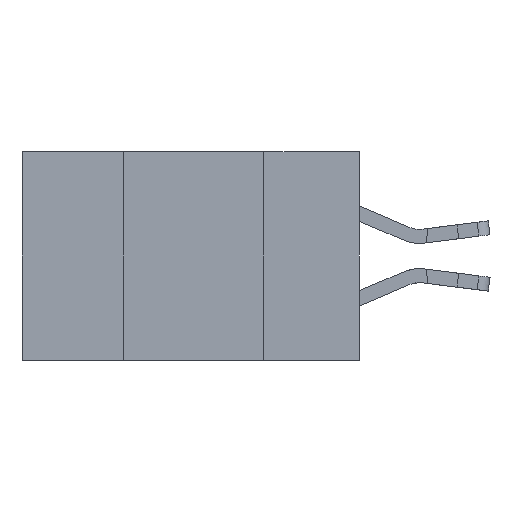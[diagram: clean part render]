
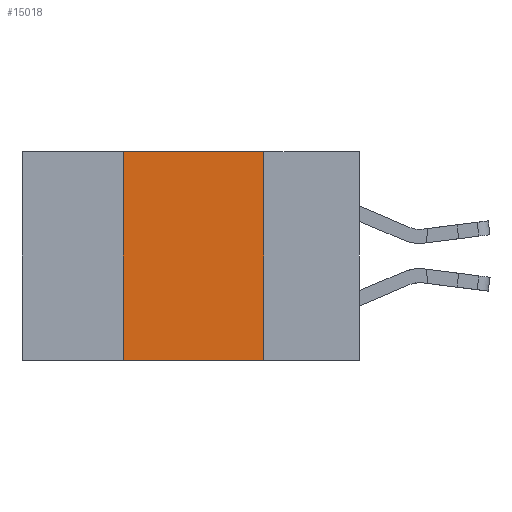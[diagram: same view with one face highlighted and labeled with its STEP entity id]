
A CAD part, left-side view. The second image highlights one B-rep face of the part: STEP entity #15018.
In plain terms, the highlighted planar face has unit normal (-1, 0, 0).
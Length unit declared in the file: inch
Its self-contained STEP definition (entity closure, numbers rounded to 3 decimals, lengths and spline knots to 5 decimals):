
#523 = AXIS2_PLACEMENT_3D ( 'NONE', #17458, #7223, #19113 ) ;
#572 = VERTEX_POINT ( 'NONE', #14570 ) ;
#1263 = CARTESIAN_POINT ( 'NONE',  ( 0., 0.17, 0. ) ) ;
#1978 = FACE_OUTER_BOUND ( 'NONE', #13921, .T. ) ;
#2129 = CARTESIAN_POINT ( 'NONE',  ( 0., 0.42, 0. ) ) ;
#2309 = CARTESIAN_POINT ( 'NONE',  ( 0., 0.42, 0. ) ) ;
#2431 = VECTOR ( 'NONE', #11048, 39.37008 ) ;
#2872 = VECTOR ( 'NONE', #20159, 39.37008 ) ;
#3584 = CARTESIAN_POINT ( 'NONE',  ( 0., 0.6, 0. ) ) ;
#5755 = VERTEX_POINT ( 'NONE', #6337 ) ;
#6337 = CARTESIAN_POINT ( 'NONE',  ( 0., 0.17, 0. ) ) ;
#6948 = DIRECTION ( 'NONE',  ( 0., -1., 0. ) ) ;
#7058 = LINE ( 'NONE', #3584, #20064 ) ;
#7223 = DIRECTION ( 'NONE',  ( 1., 0., 0. ) ) ;
#8259 = VERTEX_POINT ( 'NONE', #2129 ) ;
#8602 = EDGE_CURVE ( 'NONE', #5755, #572, #12103, .T. ) ;
#8685 = ORIENTED_EDGE ( 'NONE', *, *, #12806, .F. ) ;
#8715 = EDGE_CURVE ( 'NONE', #15789, #572, #13970, .T. ) ;
#10609 = PLANE ( 'NONE',  #523 ) ;
#10859 = ORIENTED_EDGE ( 'NONE', *, *, #18159, .F. ) ;
#11048 = DIRECTION ( 'NONE',  ( 0., 0., 1. ) ) ;
#12070 = CARTESIAN_POINT ( 'NONE',  ( 0., 0.6, -0.37 ) ) ;
#12103 = LINE ( 'NONE', #1263, #2872 ) ;
#12806 = EDGE_CURVE ( 'NONE', #8259, #5755, #7058, .T. ) ;
#13580 = ORIENTED_EDGE ( 'NONE', *, *, #8715, .T. ) ;
#13921 = EDGE_LOOP ( 'NONE', ( #15604, #8685, #10859, #13580 ) ) ;
#13970 = LINE ( 'NONE', #12070, #17935 ) ;
#14570 = CARTESIAN_POINT ( 'NONE',  ( 0., 0.17, -0.37 ) ) ;
#15018 = ADVANCED_FACE ( 'NONE', ( #1978 ), #10609, .F. ) ;
#15604 = ORIENTED_EDGE ( 'NONE', *, *, #8602, .F. ) ;
#15789 = VERTEX_POINT ( 'NONE', #21135 ) ;
#16216 = LINE ( 'NONE', #2309, #2431 ) ;
#17458 = CARTESIAN_POINT ( 'NONE',  ( 0., 0.6, 0. ) ) ;
#17935 = VECTOR ( 'NONE', #6948, 39.37008 ) ;
#18159 = EDGE_CURVE ( 'NONE', #15789, #8259, #16216, .T. ) ;
#19113 = DIRECTION ( 'NONE',  ( 0., 0., -1. ) ) ;
#20064 = VECTOR ( 'NONE', #20658, 39.37008 ) ;
#20159 = DIRECTION ( 'NONE',  ( 0., 0., -1. ) ) ;
#20658 = DIRECTION ( 'NONE',  ( 0., -1., 0. ) ) ;
#21135 = CARTESIAN_POINT ( 'NONE',  ( 0., 0.42, -0.37 ) ) ;
